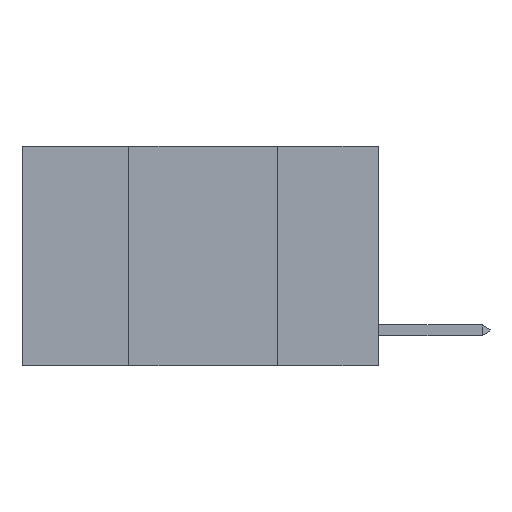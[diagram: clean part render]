
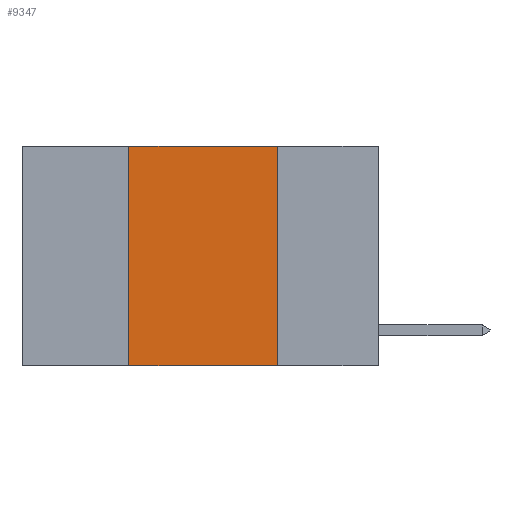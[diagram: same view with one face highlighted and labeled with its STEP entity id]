
A CAD part, left-side view. The second image highlights one B-rep face of the part: STEP entity #9347.
In plain terms, the highlighted planar face has unit normal (-1, 0, 0).
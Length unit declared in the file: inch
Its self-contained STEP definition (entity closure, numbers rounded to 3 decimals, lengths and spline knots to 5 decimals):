
#310 = DIRECTION ( 'NONE',  ( 0., 0., -1. ) ) ;
#511 = ORIENTED_EDGE ( 'NONE', *, *, #7221, .F. ) ;
#1059 = VERTEX_POINT ( 'NONE', #4748 ) ;
#1079 = CARTESIAN_POINT ( 'NONE',  ( 0., 0.6, 0. ) ) ;
#2142 = CARTESIAN_POINT ( 'NONE',  ( 0., 0.17, -0.37 ) ) ;
#2820 = CARTESIAN_POINT ( 'NONE',  ( 0., 0.42, 0. ) ) ;
#2975 = ORIENTED_EDGE ( 'NONE', *, *, #6683, .F. ) ;
#3140 = PLANE ( 'NONE',  #9657 ) ;
#3481 = CARTESIAN_POINT ( 'NONE',  ( 0., 0.6, -0.37 ) ) ;
#3691 = ORIENTED_EDGE ( 'NONE', *, *, #8702, .T. ) ;
#4271 = CARTESIAN_POINT ( 'NONE',  ( 0., 0.42, 0. ) ) ;
#4305 = CARTESIAN_POINT ( 'NONE',  ( 0., 0.6, 0. ) ) ;
#4601 = EDGE_CURVE ( 'NONE', #11191, #6945, #8308, .T. ) ;
#4748 = CARTESIAN_POINT ( 'NONE',  ( 0., 0.42, -0.37 ) ) ;
#5002 = FACE_OUTER_BOUND ( 'NONE', #13935, .T. ) ;
#5186 = CARTESIAN_POINT ( 'NONE',  ( 0., 0.17, 0. ) ) ;
#5380 = DIRECTION ( 'NONE',  ( 1., 0., 0. ) ) ;
#5773 = ORIENTED_EDGE ( 'NONE', *, *, #4601, .F. ) ;
#6683 = EDGE_CURVE ( 'NONE', #1059, #11191, #8782, .T. ) ;
#6743 = CARTESIAN_POINT ( 'NONE',  ( 0., 0.17, 0. ) ) ;
#6945 = VERTEX_POINT ( 'NONE', #5186 ) ;
#7037 = VECTOR ( 'NONE', #310, 39.37008 ) ;
#7088 = VERTEX_POINT ( 'NONE', #2142 ) ;
#7221 = EDGE_CURVE ( 'NONE', #6945, #7088, #8556, .T. ) ;
#7274 = VECTOR ( 'NONE', #9668, 39.37008 ) ;
#8214 = DIRECTION ( 'NONE',  ( 0., 0., 1. ) ) ;
#8308 = LINE ( 'NONE', #4305, #7274 ) ;
#8556 = LINE ( 'NONE', #6743, #7037 ) ;
#8702 = EDGE_CURVE ( 'NONE', #1059, #7088, #9558, .T. ) ;
#8782 = LINE ( 'NONE', #2820, #12754 ) ;
#9347 = ADVANCED_FACE ( 'NONE', ( #5002 ), #3140, .F. ) ;
#9558 = LINE ( 'NONE', #3481, #11636 ) ;
#9657 = AXIS2_PLACEMENT_3D ( 'NONE', #1079, #5380, #11839 ) ;
#9668 = DIRECTION ( 'NONE',  ( 0., -1., 0. ) ) ;
#11191 = VERTEX_POINT ( 'NONE', #4271 ) ;
#11636 = VECTOR ( 'NONE', #13233, 39.37008 ) ;
#11839 = DIRECTION ( 'NONE',  ( 0., 0., -1. ) ) ;
#12754 = VECTOR ( 'NONE', #8214, 39.37008 ) ;
#13233 = DIRECTION ( 'NONE',  ( 0., -1., 0. ) ) ;
#13935 = EDGE_LOOP ( 'NONE', ( #511, #5773, #2975, #3691 ) ) ;
